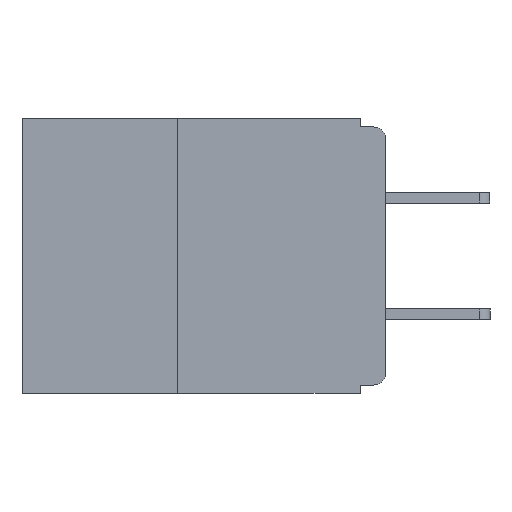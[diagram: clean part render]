
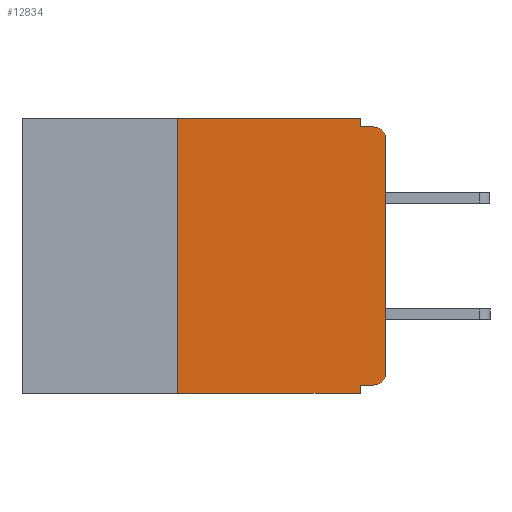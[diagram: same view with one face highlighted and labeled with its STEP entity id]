
A CAD part, left-side view. The second image highlights one B-rep face of the part: STEP entity #12834.
In plain terms, the highlighted planar face has unit normal (-1, 0, 0).
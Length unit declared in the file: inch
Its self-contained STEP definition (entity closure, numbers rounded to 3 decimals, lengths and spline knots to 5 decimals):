
#229 = LINE ( 'NONE', #7027, #17770 ) ;
#903 = ORIENTED_EDGE ( 'NONE', *, *, #8053, .F. ) ;
#1167 = EDGE_CURVE ( 'NONE', #2392, #18434, #17448, .T. ) ;
#1242 = VERTEX_POINT ( 'NONE', #14856 ) ;
#1303 = VERTEX_POINT ( 'NONE', #8389 ) ;
#1680 = AXIS2_PLACEMENT_3D ( 'NONE', #6438, #6432, #6404 ) ;
#1794 = VERTEX_POINT ( 'NONE', #21837 ) ;
#2156 = DIRECTION ( 'NONE',  ( 0., 0., -1. ) ) ;
#2392 = VERTEX_POINT ( 'NONE', #21391 ) ;
#2782 = EDGE_CURVE ( 'NONE', #5084, #1242, #3024, .T. ) ;
#2785 = CARTESIAN_POINT ( 'NONE',  ( 0., 0., -0.01 ) ) ;
#2935 = CARTESIAN_POINT ( 'NONE',  ( 0., 0., -0.32 ) ) ;
#2938 = EDGE_CURVE ( 'NONE', #20222, #3934, #17867, .T. ) ;
#2958 = ORIENTED_EDGE ( 'NONE', *, *, #18682, .F. ) ;
#2975 = LINE ( 'NONE', #17455, #11523 ) ;
#3024 = LINE ( 'NONE', #15344, #7504 ) ;
#3658 = ORIENTED_EDGE ( 'NONE', *, *, #2938, .T. ) ;
#3904 = VECTOR ( 'NONE', #5391, 39.37008 ) ;
#3934 = VERTEX_POINT ( 'NONE', #19520 ) ;
#4056 = ORIENTED_EDGE ( 'NONE', *, *, #12513, .F. ) ;
#5084 = VERTEX_POINT ( 'NONE', #12073 ) ;
#5391 = DIRECTION ( 'NONE',  ( 0., -1., 0. ) ) ;
#5440 = EDGE_CURVE ( 'NONE', #1242, #18434, #20848, .T. ) ;
#6335 = DIRECTION ( 'NONE',  ( 0., -1., 0. ) ) ;
#6404 = DIRECTION ( 'NONE',  ( 0., 0., -1. ) ) ;
#6432 = DIRECTION ( 'NONE',  ( -1., 0., 0. ) ) ;
#6438 = CARTESIAN_POINT ( 'NONE',  ( 0., 0.015, -0.025 ) ) ;
#7027 = CARTESIAN_POINT ( 'NONE',  ( 0., 0.031, 0. ) ) ;
#7231 = VECTOR ( 'NONE', #14913, 39.37008 ) ;
#7504 = VECTOR ( 'NONE', #15882, 39.37008 ) ;
#7558 = CARTESIAN_POINT ( 'NONE',  ( 0., 0.015, -0.305 ) ) ;
#7600 = LINE ( 'NONE', #16595, #11678 ) ;
#8053 = EDGE_CURVE ( 'NONE', #9447, #3934, #2975, .T. ) ;
#8389 = CARTESIAN_POINT ( 'NONE',  ( 0., 0.25, 0. ) ) ;
#8860 = VECTOR ( 'NONE', #6335, 39.37008 ) ;
#9263 = VECTOR ( 'NONE', #10063, 39.37008 ) ;
#9304 = DIRECTION ( 'NONE',  ( 0., 0., -1. ) ) ;
#9447 = VERTEX_POINT ( 'NONE', #10111 ) ;
#9799 = LINE ( 'NONE', #20132, #9263 ) ;
#10063 = DIRECTION ( 'NONE',  ( 0., -1., 0. ) ) ;
#10111 = CARTESIAN_POINT ( 'NONE',  ( 0., 0.031, -0.32 ) ) ;
#11399 = CARTESIAN_POINT ( 'NONE',  ( 0., 0.437, 0. ) ) ;
#11469 = DIRECTION ( 'NONE',  ( 0., 0., -1. ) ) ;
#11523 = VECTOR ( 'NONE', #2156, 39.37008 ) ;
#11678 = VECTOR ( 'NONE', #14949, 39.37008 ) ;
#12073 = CARTESIAN_POINT ( 'NONE',  ( 0., 0., -0.305 ) ) ;
#12096 = CIRCLE ( 'NONE', #19752, 0.015 ) ;
#12373 = LINE ( 'NONE', #2935, #7231 ) ;
#12513 = EDGE_CURVE ( 'NONE', #21534, #2392, #229, .T. ) ;
#12610 = ORIENTED_EDGE ( 'NONE', *, *, #16886, .T. ) ;
#12834 = ADVANCED_FACE ( 'NONE', ( #15985 ), #19818, .F. ) ;
#13933 = ORIENTED_EDGE ( 'NONE', *, *, #21599, .F. ) ;
#14692 = CARTESIAN_POINT ( 'NONE',  ( 0., 0.031, 0. ) ) ;
#14856 = CARTESIAN_POINT ( 'NONE',  ( 0., 0., -0.025 ) ) ;
#14901 = EDGE_LOOP ( 'NONE', ( #15290, #17901, #21162, #4056, #21453, #2958, #3658, #903, #13933, #12610 ) ) ;
#14913 = DIRECTION ( 'NONE',  ( 0., 1., 0. ) ) ;
#14949 = DIRECTION ( 'NONE',  ( 0., 0., 1. ) ) ;
#15290 = ORIENTED_EDGE ( 'NONE', *, *, #2782, .T. ) ;
#15344 = CARTESIAN_POINT ( 'NONE',  ( 0., 0., 0. ) ) ;
#15609 = DIRECTION ( 'NONE',  ( 0., 0., -1. ) ) ;
#15882 = DIRECTION ( 'NONE',  ( 0., 0., 1. ) ) ;
#15966 = CARTESIAN_POINT ( 'NONE',  ( 0., 0.437, -0.33 ) ) ;
#15985 = FACE_OUTER_BOUND ( 'NONE', #14901, .T. ) ;
#16595 = CARTESIAN_POINT ( 'NONE',  ( 0., 0.25, -0.33 ) ) ;
#16886 = EDGE_CURVE ( 'NONE', #1794, #5084, #12096, .T. ) ;
#17448 = LINE ( 'NONE', #2785, #3904 ) ;
#17455 = CARTESIAN_POINT ( 'NONE',  ( 0., 0.031, -0.33 ) ) ;
#17479 = AXIS2_PLACEMENT_3D ( 'NONE', #11399, #21452, #11469 ) ;
#17770 = VECTOR ( 'NONE', #15609, 39.37008 ) ;
#17867 = LINE ( 'NONE', #15966, #8860 ) ;
#17901 = ORIENTED_EDGE ( 'NONE', *, *, #5440, .T. ) ;
#18124 = EDGE_CURVE ( 'NONE', #1303, #21534, #9799, .T. ) ;
#18434 = VERTEX_POINT ( 'NONE', #19277 ) ;
#18682 = EDGE_CURVE ( 'NONE', #20222, #1303, #7600, .T. ) ;
#19277 = CARTESIAN_POINT ( 'NONE',  ( 0., 0.015, -0.01 ) ) ;
#19425 = DIRECTION ( 'NONE',  ( -1., 0., 0. ) ) ;
#19520 = CARTESIAN_POINT ( 'NONE',  ( 0., 0.031, -0.33 ) ) ;
#19752 = AXIS2_PLACEMENT_3D ( 'NONE', #7558, #19425, #9304 ) ;
#19818 = PLANE ( 'NONE',  #17479 ) ;
#20132 = CARTESIAN_POINT ( 'NONE',  ( 0., 0.437, 0. ) ) ;
#20222 = VERTEX_POINT ( 'NONE', #20771 ) ;
#20771 = CARTESIAN_POINT ( 'NONE',  ( 0., 0.25, -0.33 ) ) ;
#20848 = CIRCLE ( 'NONE', #1680, 0.015 ) ;
#21162 = ORIENTED_EDGE ( 'NONE', *, *, #1167, .F. ) ;
#21391 = CARTESIAN_POINT ( 'NONE',  ( 0., 0.031, -0.01 ) ) ;
#21452 = DIRECTION ( 'NONE',  ( 1., 0., 0. ) ) ;
#21453 = ORIENTED_EDGE ( 'NONE', *, *, #18124, .F. ) ;
#21534 = VERTEX_POINT ( 'NONE', #14692 ) ;
#21599 = EDGE_CURVE ( 'NONE', #1794, #9447, #12373, .T. ) ;
#21837 = CARTESIAN_POINT ( 'NONE',  ( 0., 0.015, -0.32 ) ) ;
